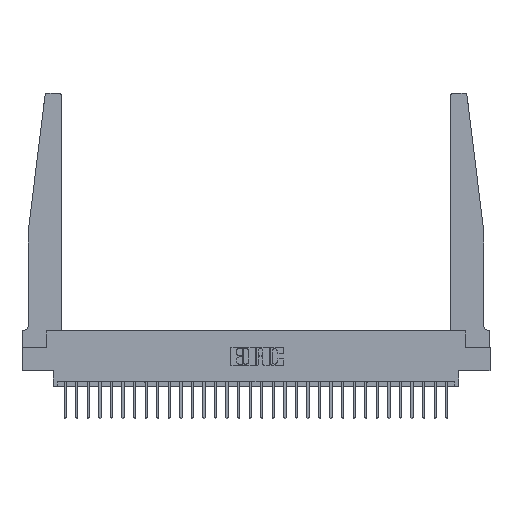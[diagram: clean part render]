
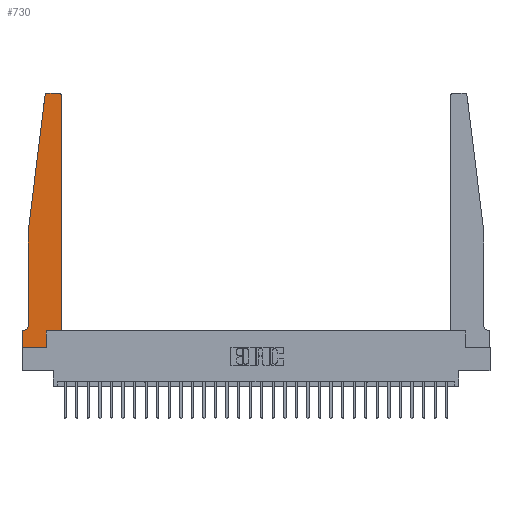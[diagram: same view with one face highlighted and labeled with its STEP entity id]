
A CAD part, top view. The second image highlights one B-rep face of the part: STEP entity #730.
In plain terms, the highlighted planar face has unit normal (0, 0, 1).
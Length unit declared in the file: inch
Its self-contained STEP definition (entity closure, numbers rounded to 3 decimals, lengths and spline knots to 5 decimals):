
#133 = DIRECTION ( 'NONE',  ( -1., 0., 0. ) ) ;
#454 = DIRECTION ( 'NONE',  ( 1., 0., 0. ) ) ;
#459 = CARTESIAN_POINT ( 'NONE',  ( 0.425, 0.18, 0.37 ) ) ;
#730 = ADVANCED_FACE ( 'NONE', ( #27649 ), #26574, .T. ) ;
#787 = EDGE_CURVE ( 'NONE', #20057, #25255, #19162, .T. ) ;
#1244 = VECTOR ( 'NONE', #21163, 39.37008 ) ;
#1279 = EDGE_CURVE ( 'NONE', #20721, #2672, #20497, .T. ) ;
#1697 = CARTESIAN_POINT ( 'NONE',  ( 0., 0., 0.37 ) ) ;
#2290 = CARTESIAN_POINT ( 'NONE',  ( 0.065, 1.25, 0.37 ) ) ;
#2540 = EDGE_CURVE ( 'NONE', #11748, #27170, #12929, .T. ) ;
#2672 = VERTEX_POINT ( 'NONE', #20210 ) ;
#2742 = CIRCLE ( 'NONE', #19070, 0.05 ) ;
#2979 = CARTESIAN_POINT ( 'NONE',  ( 0., 0.1875, 0.37 ) ) ;
#3300 = VECTOR ( 'NONE', #22287, 39.37008 ) ;
#4800 = DIRECTION ( 'NONE',  ( 0., 0., 1. ) ) ;
#4827 = VECTOR ( 'NONE', #13195, 39.37008 ) ;
#5077 = CARTESIAN_POINT ( 'NONE',  ( 0., 0., 0.37 ) ) ;
#5427 = VECTOR ( 'NONE', #10191, 39.37008 ) ;
#5560 = ORIENTED_EDGE ( 'NONE', *, *, #2540, .T. ) ;
#5613 = ORIENTED_EDGE ( 'NONE', *, *, #10995, .T. ) ;
#5940 = VERTEX_POINT ( 'NONE', #22261 ) ;
#7205 = DIRECTION ( 'NONE',  ( 0., 0., 1. ) ) ;
#7285 = DIRECTION ( 'NONE',  ( 1., 0., 0. ) ) ;
#7359 = CARTESIAN_POINT ( 'NONE',  ( 0.065, 0.2375, 0.37 ) ) ;
#7571 = VECTOR ( 'NONE', #7285, 39.37008 ) ;
#8036 = VERTEX_POINT ( 'NONE', #7359 ) ;
#8064 = CARTESIAN_POINT ( 'NONE',  ( 0.2605, 0.18, 0.37 ) ) ;
#8516 = VERTEX_POINT ( 'NONE', #8064 ) ;
#8863 = CARTESIAN_POINT ( 'NONE',  ( 0.25, 2.75, 0.37 ) ) ;
#9186 = VECTOR ( 'NONE', #15400, 39.37008 ) ;
#9703 = VECTOR ( 'NONE', #19213, 39.37008 ) ;
#10002 = ORIENTED_EDGE ( 'NONE', *, *, #1279, .T. ) ;
#10191 = DIRECTION ( 'NONE',  ( -1., 0., 0. ) ) ;
#10296 = EDGE_CURVE ( 'NONE', #5940, #13984, #22764, .T. ) ;
#10350 = CARTESIAN_POINT ( 'NONE',  ( 0.2605, 0.18, 0.37 ) ) ;
#10705 = CARTESIAN_POINT ( 'NONE',  ( 0.015, 0.2375, 0.37 ) ) ;
#10995 = EDGE_CURVE ( 'NONE', #25255, #8516, #18670, .T. ) ;
#11032 = CARTESIAN_POINT ( 'NONE',  ( 0.425, 0.18, 0.37 ) ) ;
#11037 = AXIS2_PLACEMENT_3D ( 'NONE', #20236, #7205, #22391 ) ;
#11364 = ORIENTED_EDGE ( 'NONE', *, *, #20106, .T. ) ;
#11448 = EDGE_LOOP ( 'NONE', ( #10002, #20939, #5560, #26707, #11364, #22273, #17184, #17841, #5613, #23589, #12087, #19205 ) ) ;
#11748 = VERTEX_POINT ( 'NONE', #19659 ) ;
#12087 = ORIENTED_EDGE ( 'NONE', *, *, #14478, .T. ) ;
#12262 = CARTESIAN_POINT ( 'NONE',  ( 0.2605, 0., 0.37 ) ) ;
#12283 = DIRECTION ( 'NONE',  ( 0., 0., 1. ) ) ;
#12871 = DIRECTION ( 'NONE',  ( -1., 0., 0. ) ) ;
#12929 = LINE ( 'NONE', #2290, #9186 ) ;
#13002 = CIRCLE ( 'NONE', #11037, 0.03 ) ;
#13195 = DIRECTION ( 'NONE',  ( 1., 0., 0. ) ) ;
#13826 = CARTESIAN_POINT ( 'NONE',  ( 0.065, 1.25, 0.37 ) ) ;
#13984 = VERTEX_POINT ( 'NONE', #2979 ) ;
#14478 = EDGE_CURVE ( 'NONE', #18406, #18350, #15624, .T. ) ;
#14936 = CARTESIAN_POINT ( 'NONE',  ( 0.425, 0.18, 0.37 ) ) ;
#15400 = DIRECTION ( 'NONE',  ( -0.122, -0.992, 0. ) ) ;
#15537 = AXIS2_PLACEMENT_3D ( 'NONE', #25281, #12283, #27480 ) ;
#15624 = LINE ( 'NONE', #459, #3300 ) ;
#16946 = CARTESIAN_POINT ( 'NONE',  ( 0.425, 2.72, 0.37 ) ) ;
#16967 = CARTESIAN_POINT ( 'NONE',  ( 0.395, 2.75, 0.37 ) ) ;
#17184 = ORIENTED_EDGE ( 'NONE', *, *, #25411, .T. ) ;
#17841 = ORIENTED_EDGE ( 'NONE', *, *, #787, .T. ) ;
#18350 = VERTEX_POINT ( 'NONE', #16946 ) ;
#18406 = VERTEX_POINT ( 'NONE', #14936 ) ;
#18528 = EDGE_CURVE ( 'NONE', #8516, #18406, #22175, .T. ) ;
#18652 = EDGE_CURVE ( 'NONE', #18350, #20721, #13002, .T. ) ;
#18670 = LINE ( 'NONE', #10350, #1244 ) ;
#19070 = AXIS2_PLACEMENT_3D ( 'NONE', #10705, #25901, #12871 ) ;
#19162 = LINE ( 'NONE', #5077, #7571 ) ;
#19205 = ORIENTED_EDGE ( 'NONE', *, *, #18652, .T. ) ;
#19213 = DIRECTION ( 'NONE',  ( 0., -1., 0. ) ) ;
#19659 = CARTESIAN_POINT ( 'NONE',  ( 0.24675, 2.72367, 0.37 ) ) ;
#20057 = VERTEX_POINT ( 'NONE', #1697 ) ;
#20106 = EDGE_CURVE ( 'NONE', #8036, #5940, #2742, .T. ) ;
#20210 = CARTESIAN_POINT ( 'NONE',  ( 0.27653, 2.75, 0.37 ) ) ;
#20236 = CARTESIAN_POINT ( 'NONE',  ( 0.395, 2.72, 0.37 ) ) ;
#20497 = LINE ( 'NONE', #8863, #25573 ) ;
#20721 = VERTEX_POINT ( 'NONE', #16967 ) ;
#20939 = ORIENTED_EDGE ( 'NONE', *, *, #27372, .T. ) ;
#21014 = CARTESIAN_POINT ( 'NONE',  ( 0.065, 0.1875, 0.37 ) ) ;
#21163 = DIRECTION ( 'NONE',  ( 0., 1., 0. ) ) ;
#21474 = CARTESIAN_POINT ( 'NONE',  ( 0.065, 1.25, 0.37 ) ) ;
#21905 = CIRCLE ( 'NONE', #15537, 0.03 ) ;
#22175 = LINE ( 'NONE', #11032, #4827 ) ;
#22261 = CARTESIAN_POINT ( 'NONE',  ( 0.015, 0.1875, 0.37 ) ) ;
#22273 = ORIENTED_EDGE ( 'NONE', *, *, #10296, .T. ) ;
#22287 = DIRECTION ( 'NONE',  ( 0., 1., 0. ) ) ;
#22391 = DIRECTION ( 'NONE',  ( 1., 0., 0. ) ) ;
#22764 = LINE ( 'NONE', #21014, #5427 ) ;
#22938 = AXIS2_PLACEMENT_3D ( 'NONE', #24385, #4800, #454 ) ;
#23553 = CARTESIAN_POINT ( 'NONE',  ( 0., 0., 0.37 ) ) ;
#23589 = ORIENTED_EDGE ( 'NONE', *, *, #18528, .T. ) ;
#23629 = DIRECTION ( 'NONE',  ( 0., -1., 0. ) ) ;
#24385 = CARTESIAN_POINT ( 'NONE',  ( 0., 0.1875, 0.37 ) ) ;
#25255 = VERTEX_POINT ( 'NONE', #12262 ) ;
#25281 = CARTESIAN_POINT ( 'NONE',  ( 0.27653, 2.72, 0.37 ) ) ;
#25411 = EDGE_CURVE ( 'NONE', #13984, #20057, #27705, .T. ) ;
#25573 = VECTOR ( 'NONE', #133, 39.37008 ) ;
#25901 = DIRECTION ( 'NONE',  ( 0., 0., -1. ) ) ;
#25950 = VECTOR ( 'NONE', #23629, 39.37008 ) ;
#26574 = PLANE ( 'NONE',  #22938 ) ;
#26623 = LINE ( 'NONE', #21474, #25950 ) ;
#26707 = ORIENTED_EDGE ( 'NONE', *, *, #28188, .T. ) ;
#27170 = VERTEX_POINT ( 'NONE', #13826 ) ;
#27372 = EDGE_CURVE ( 'NONE', #2672, #11748, #21905, .T. ) ;
#27480 = DIRECTION ( 'NONE',  ( 1., 0., 0. ) ) ;
#27649 = FACE_OUTER_BOUND ( 'NONE', #11448, .T. ) ;
#27705 = LINE ( 'NONE', #23553, #9703 ) ;
#28188 = EDGE_CURVE ( 'NONE', #27170, #8036, #26623, .T. ) ;
